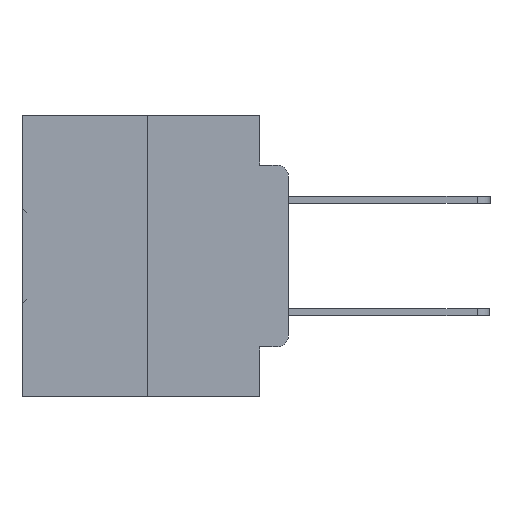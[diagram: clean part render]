
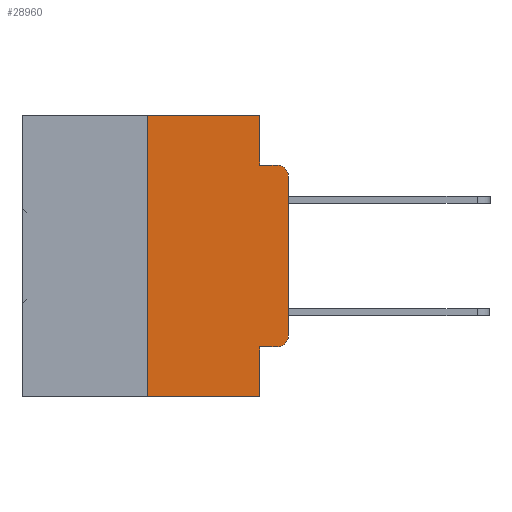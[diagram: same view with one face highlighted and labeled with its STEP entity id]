
A CAD part, left-side view. The second image highlights one B-rep face of the part: STEP entity #28960.
In plain terms, the highlighted planar face has unit normal (-1, 0, 0).
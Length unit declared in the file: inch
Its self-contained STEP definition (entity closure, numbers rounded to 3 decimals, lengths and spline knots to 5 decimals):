
#278 = VECTOR ( 'NONE', #18926, 39.37008 ) ;
#629 = CARTESIAN_POINT ( 'NONE',  ( 0., 0.051, -0.0885 ) ) ;
#987 = EDGE_CURVE ( 'NONE', #16941, #3424, #7664, .T. ) ;
#1409 = FACE_OUTER_BOUND ( 'NONE', #25119, .T. ) ;
#2002 = VERTEX_POINT ( 'NONE', #27780 ) ;
#2287 = VECTOR ( 'NONE', #28984, 39.37008 ) ;
#2389 = VERTEX_POINT ( 'NONE', #22318 ) ;
#2535 = VECTOR ( 'NONE', #11238, 39.37008 ) ;
#3424 = VERTEX_POINT ( 'NONE', #8370 ) ;
#3494 = DIRECTION ( 'NONE',  ( 0., -1., 0. ) ) ;
#3739 = VERTEX_POINT ( 'NONE', #9904 ) ;
#3835 = ORIENTED_EDGE ( 'NONE', *, *, #9630, .F. ) ;
#4711 = CARTESIAN_POINT ( 'NONE',  ( 0., 0.02, -0.1085 ) ) ;
#5969 = VERTEX_POINT ( 'NONE', #22432 ) ;
#6008 = LINE ( 'NONE', #21077, #20854 ) ;
#7469 = DIRECTION ( 'NONE',  ( 0., 0., -1. ) ) ;
#7664 = LINE ( 'NONE', #18753, #278 ) ;
#7932 = CARTESIAN_POINT ( 'NONE',  ( 0., 0.25, -0.5 ) ) ;
#8370 = CARTESIAN_POINT ( 'NONE',  ( 0., 0.02, -0.0885 ) ) ;
#8746 = CARTESIAN_POINT ( 'NONE',  ( 0., 0.02, -0.4115 ) ) ;
#8958 = ORIENTED_EDGE ( 'NONE', *, *, #22075, .F. ) ;
#9630 = EDGE_CURVE ( 'NONE', #14018, #3739, #6008, .T. ) ;
#9904 = CARTESIAN_POINT ( 'NONE',  ( 0., 0.25, 0. ) ) ;
#11099 = ORIENTED_EDGE ( 'NONE', *, *, #18273, .T. ) ;
#11238 = DIRECTION ( 'NONE',  ( 0., -1., 0. ) ) ;
#11603 = EDGE_CURVE ( 'NONE', #2002, #3424, #13590, .T. ) ;
#11926 = ORIENTED_EDGE ( 'NONE', *, *, #987, .F. ) ;
#12290 = CARTESIAN_POINT ( 'NONE',  ( 0., 0., 0. ) ) ;
#12846 = EDGE_CURVE ( 'NONE', #5969, #16941, #31708, .T. ) ;
#13075 = VECTOR ( 'NONE', #26130, 39.37008 ) ;
#13570 = DIRECTION ( 'NONE',  ( 0., -1., 0. ) ) ;
#13590 = CIRCLE ( 'NONE', #25442, 0.02 ) ;
#13962 = LINE ( 'NONE', #28865, #13075 ) ;
#14018 = VERTEX_POINT ( 'NONE', #7932 ) ;
#14222 = CARTESIAN_POINT ( 'NONE',  ( 0., 0.02, -0.3915 ) ) ;
#14477 = CARTESIAN_POINT ( 'NONE',  ( 0., 0.051, -0.4115 ) ) ;
#15739 = EDGE_CURVE ( 'NONE', #2389, #2002, #25359, .T. ) ;
#15895 = DIRECTION ( 'NONE',  ( 1., 0., 0. ) ) ;
#16703 = AXIS2_PLACEMENT_3D ( 'NONE', #26969, #15895, #35140 ) ;
#16933 = CARTESIAN_POINT ( 'NONE',  ( 0., 0.051, -0.5 ) ) ;
#16941 = VERTEX_POINT ( 'NONE', #629 ) ;
#17099 = DIRECTION ( 'NONE',  ( 0., 0., -1. ) ) ;
#18234 = LINE ( 'NONE', #33394, #2535 ) ;
#18273 = EDGE_CURVE ( 'NONE', #14018, #18321, #18234, .T. ) ;
#18321 = VERTEX_POINT ( 'NONE', #16933 ) ;
#18753 = CARTESIAN_POINT ( 'NONE',  ( 0., 0.051, -0.0885 ) ) ;
#18926 = DIRECTION ( 'NONE',  ( 0., -1., 0. ) ) ;
#19060 = ORIENTED_EDGE ( 'NONE', *, *, #19602, .T. ) ;
#19490 = ORIENTED_EDGE ( 'NONE', *, *, #12846, .F. ) ;
#19602 = EDGE_CURVE ( 'NONE', #20179, #2389, #27215, .T. ) ;
#20179 = VERTEX_POINT ( 'NONE', #8746 ) ;
#20267 = LINE ( 'NONE', #14477, #33911 ) ;
#20406 = ORIENTED_EDGE ( 'NONE', *, *, #29269, .F. ) ;
#20854 = VECTOR ( 'NONE', #23865, 39.37008 ) ;
#21077 = CARTESIAN_POINT ( 'NONE',  ( 0., 0.25, 0. ) ) ;
#21845 = DIRECTION ( 'NONE',  ( 0., 0., -1. ) ) ;
#22075 = EDGE_CURVE ( 'NONE', #3739, #5969, #26475, .T. ) ;
#22318 = CARTESIAN_POINT ( 'NONE',  ( 0., 0., -0.3915 ) ) ;
#22432 = CARTESIAN_POINT ( 'NONE',  ( 0., 0.051, 0. ) ) ;
#23865 = DIRECTION ( 'NONE',  ( 0., 0., 1. ) ) ;
#24219 = DIRECTION ( 'NONE',  ( -1., 0., 0. ) ) ;
#24499 = EDGE_CURVE ( 'NONE', #28861, #20179, #20267, .T. ) ;
#24512 = VECTOR ( 'NONE', #21845, 39.37008 ) ;
#25119 = EDGE_LOOP ( 'NONE', ( #29333, #31490, #11926, #19490, #8958, #3835, #11099, #20406, #27718, #19060 ) ) ;
#25359 = LINE ( 'NONE', #12290, #2287 ) ;
#25442 = AXIS2_PLACEMENT_3D ( 'NONE', #4711, #24219, #7469 ) ;
#26130 = DIRECTION ( 'NONE',  ( 0., 0., -1. ) ) ;
#26475 = LINE ( 'NONE', #30218, #33682 ) ;
#26969 = CARTESIAN_POINT ( 'NONE',  ( 0., 0.473, 0. ) ) ;
#27215 = CIRCLE ( 'NONE', #28574, 0.02 ) ;
#27718 = ORIENTED_EDGE ( 'NONE', *, *, #24499, .T. ) ;
#27780 = CARTESIAN_POINT ( 'NONE',  ( 0., 0., -0.1085 ) ) ;
#28574 = AXIS2_PLACEMENT_3D ( 'NONE', #14222, #33553, #17099 ) ;
#28861 = VERTEX_POINT ( 'NONE', #34668 ) ;
#28865 = CARTESIAN_POINT ( 'NONE',  ( 0., 0.051, 0. ) ) ;
#28960 = ADVANCED_FACE ( 'NONE', ( #1409 ), #32406, .F. ) ;
#28984 = DIRECTION ( 'NONE',  ( 0., 0., 1. ) ) ;
#29269 = EDGE_CURVE ( 'NONE', #28861, #18321, #13962, .T. ) ;
#29333 = ORIENTED_EDGE ( 'NONE', *, *, #15739, .T. ) ;
#30218 = CARTESIAN_POINT ( 'NONE',  ( 0., 0.473, 0. ) ) ;
#31490 = ORIENTED_EDGE ( 'NONE', *, *, #11603, .T. ) ;
#31708 = LINE ( 'NONE', #32655, #24512 ) ;
#32406 = PLANE ( 'NONE',  #16703 ) ;
#32655 = CARTESIAN_POINT ( 'NONE',  ( 0., 0.051, 0. ) ) ;
#33394 = CARTESIAN_POINT ( 'NONE',  ( 0., 0.473, -0.5 ) ) ;
#33553 = DIRECTION ( 'NONE',  ( -1., 0., 0. ) ) ;
#33682 = VECTOR ( 'NONE', #13570, 39.37008 ) ;
#33911 = VECTOR ( 'NONE', #3494, 39.37008 ) ;
#34668 = CARTESIAN_POINT ( 'NONE',  ( 0., 0.051, -0.4115 ) ) ;
#35140 = DIRECTION ( 'NONE',  ( 0., 0., -1. ) ) ;
